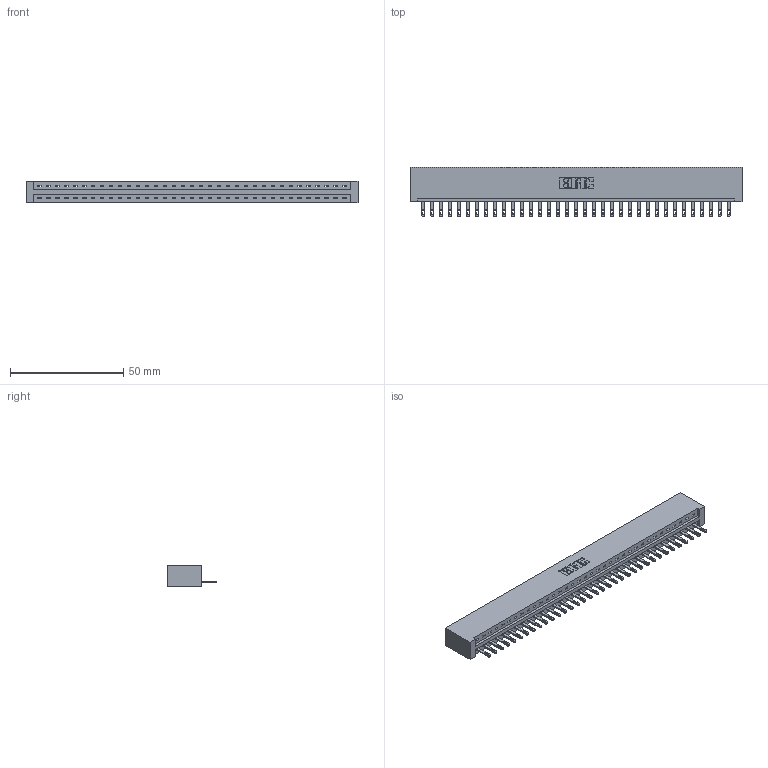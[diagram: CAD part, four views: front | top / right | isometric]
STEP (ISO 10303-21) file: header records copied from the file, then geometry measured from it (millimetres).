
FILE_DESCRIPTION (( 'STEP AP203' ), '1' );
FILE_NAME ('887-035-500-101.STEP', '2020-09-20T21:53:57', ( '' ), ( '' ), 'SwSTEP 2.0', 'SolidWorks 2020', '' );
FILE_SCHEMA (( 'CONFIG_CONTROL_DESIGN' ));
Length unit declared in the file: inch
Products named in the file (3): 345-292-001_345-293-100; 887-035-500-101; 837 Part_No Mounting Lugs
Assembly tree (36 placements, depth 2):
  887-035-500-101
    837 Part_No Mounting Lugs
    345-292-001_345-293-100  x35
Bounding box: 146.56 x 21.85 x 9.4 mm (x, y, z)
Volume: 15905 mm3; surface area: 16459.8 mm2
Topology: 36 solids, 36 shells, 2136 faces, 6587 edges, 4390 vertices
Faces by surface type: plane 1466, cylinder 670
Entity records: 26575 total; most frequent: CARTESIAN_POINT 4635, ORIENTED_EDGE 4606, DIRECTION 3909, EDGE_CURVE 2303, LINE 2179, VECTOR 2179, VERTEX_POINT 1534, AXIS2_PLACEMENT_3D 865
